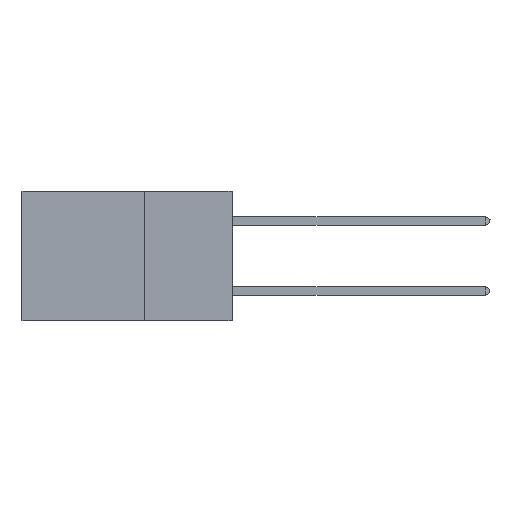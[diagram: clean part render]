
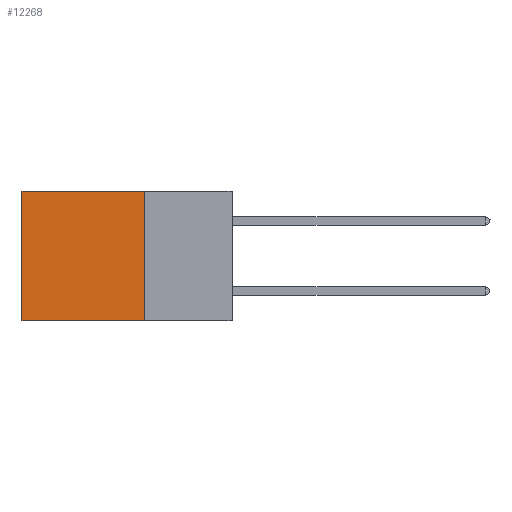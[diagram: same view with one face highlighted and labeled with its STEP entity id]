
A CAD part, left-side view. The second image highlights one B-rep face of the part: STEP entity #12268.
In plain terms, the highlighted planar face has unit normal (-1, 0, 0).
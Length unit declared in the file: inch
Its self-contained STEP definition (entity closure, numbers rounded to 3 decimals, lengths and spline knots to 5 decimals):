
#1372 = VERTEX_POINT ( 'NONE', #17673 ) ;
#1484 = EDGE_CURVE ( 'NONE', #14611, #1606, #20869, .T. ) ;
#1606 = VERTEX_POINT ( 'NONE', #24353 ) ;
#3127 = EDGE_CURVE ( 'NONE', #1372, #10056, #20145, .T. ) ;
#3660 = EDGE_LOOP ( 'NONE', ( #6665, #22984, #13564, #21910 ) ) ;
#4361 = CARTESIAN_POINT ( 'NONE',  ( 0.2875, 0.25, -0.37 ) ) ;
#5075 = VECTOR ( 'NONE', #16115, 39.37008 ) ;
#5232 = VECTOR ( 'NONE', #14205, 39.37008 ) ;
#5432 = CARTESIAN_POINT ( 'NONE',  ( 0.2875, 0.25, 0. ) ) ;
#6492 = LINE ( 'NONE', #4361, #5232 ) ;
#6509 = CARTESIAN_POINT ( 'NONE',  ( 0.2875, 0.6, 0. ) ) ;
#6665 = ORIENTED_EDGE ( 'NONE', *, *, #1484, .T. ) ;
#8590 = CARTESIAN_POINT ( 'NONE',  ( 0.2875, 0.25, 0. ) ) ;
#8999 = VECTOR ( 'NONE', #14674, 39.37008 ) ;
#9984 = CARTESIAN_POINT ( 'NONE',  ( 0.2875, 0.25, -0.37 ) ) ;
#10056 = VERTEX_POINT ( 'NONE', #9984 ) ;
#10579 = DIRECTION ( 'NONE',  ( 0., 0., -1. ) ) ;
#12268 = ADVANCED_FACE ( 'NONE', ( #14669 ), #18482, .F. ) ;
#13564 = ORIENTED_EDGE ( 'NONE', *, *, #3127, .F. ) ;
#14205 = DIRECTION ( 'NONE',  ( 0., 1., 0. ) ) ;
#14611 = VERTEX_POINT ( 'NONE', #6509 ) ;
#14669 = FACE_OUTER_BOUND ( 'NONE', #3660, .T. ) ;
#14674 = DIRECTION ( 'NONE',  ( 0., 0., -1. ) ) ;
#14767 = CARTESIAN_POINT ( 'NONE',  ( 0.2875, 0.25, 0. ) ) ;
#15200 = LINE ( 'NONE', #5432, #20430 ) ;
#15209 = EDGE_CURVE ( 'NONE', #10056, #1606, #6492, .T. ) ;
#16115 = DIRECTION ( 'NONE',  ( 0., 0., -1. ) ) ;
#17673 = CARTESIAN_POINT ( 'NONE',  ( 0.2875, 0.25, 0. ) ) ;
#18110 = CARTESIAN_POINT ( 'NONE',  ( 0.2875, 0.6, 0. ) ) ;
#18482 = PLANE ( 'NONE',  #24982 ) ;
#19288 = DIRECTION ( 'NONE',  ( 0., 1., 0. ) ) ;
#20145 = LINE ( 'NONE', #14767, #8999 ) ;
#20430 = VECTOR ( 'NONE', #19288, 39.37008 ) ;
#20869 = LINE ( 'NONE', #18110, #5075 ) ;
#21910 = ORIENTED_EDGE ( 'NONE', *, *, #24089, .T. ) ;
#22412 = DIRECTION ( 'NONE',  ( 1., 0., 0. ) ) ;
#22984 = ORIENTED_EDGE ( 'NONE', *, *, #15209, .F. ) ;
#24089 = EDGE_CURVE ( 'NONE', #1372, #14611, #15200, .T. ) ;
#24353 = CARTESIAN_POINT ( 'NONE',  ( 0.2875, 0.6, -0.37 ) ) ;
#24982 = AXIS2_PLACEMENT_3D ( 'NONE', #8590, #22412, #10579 ) ;
